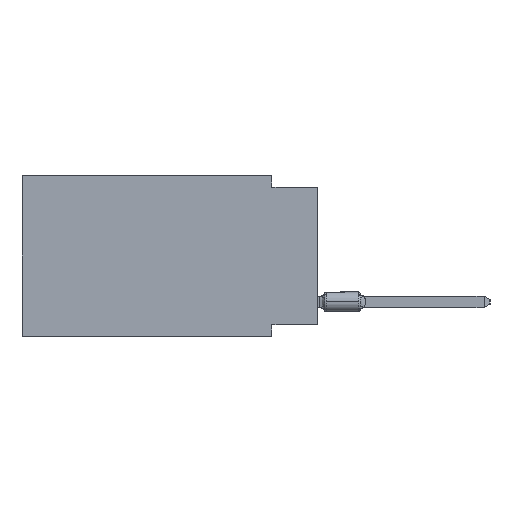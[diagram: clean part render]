
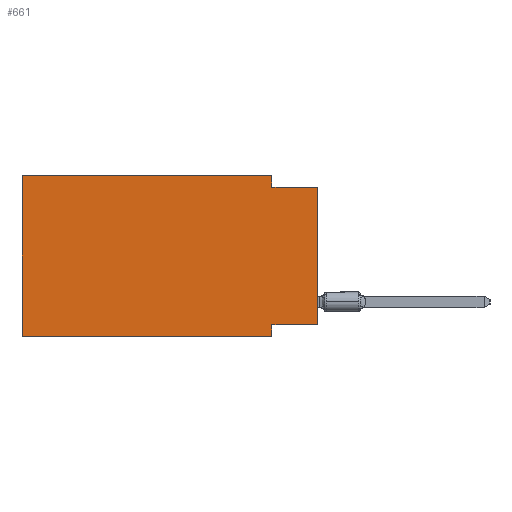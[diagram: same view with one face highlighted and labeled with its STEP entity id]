
A CAD part, left-side view. The second image highlights one B-rep face of the part: STEP entity #661.
In plain terms, the highlighted planar face has unit normal (-1, 0, 0).
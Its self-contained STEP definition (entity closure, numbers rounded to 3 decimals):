
#661 = ADVANCED_FACE ( 'NONE', ( #26702 ), #38116, .F. ) ;
#1163 = LINE ( 'NONE', #56208, #45565 ) ;
#1290 = VECTOR ( 'NONE', #16226, 1000. ) ;
#2733 = CARTESIAN_POINT ( 'NONE',  ( 0., 16.383, 0. ) ) ;
#2966 = CARTESIAN_POINT ( 'NONE',  ( 0., 16.383, 0. ) ) ;
#3619 = DIRECTION ( 'NONE',  ( 0., 0., 1. ) ) ;
#6558 = CARTESIAN_POINT ( 'NONE',  ( 0., 2.54, -0.635 ) ) ;
#6647 = LINE ( 'NONE', #50279, #53471 ) ;
#6813 = VERTEX_POINT ( 'NONE', #57139 ) ;
#7743 = LINE ( 'NONE', #2733, #22781 ) ;
#8327 = DIRECTION ( 'NONE',  ( 0., 1., 0. ) ) ;
#9110 = CARTESIAN_POINT ( 'NONE',  ( 0., 2.54, -8.89 ) ) ;
#10935 = CARTESIAN_POINT ( 'NONE',  ( 0., 16.383, -8.89 ) ) ;
#11896 = DIRECTION ( 'NONE',  ( 0., -1., 0. ) ) ;
#14308 = EDGE_CURVE ( 'NONE', #36126, #22864, #6647, .T. ) ;
#14360 = LINE ( 'NONE', #18653, #56139 ) ;
#15559 = ORIENTED_EDGE ( 'NONE', *, *, #39567, .T. ) ;
#16226 = DIRECTION ( 'NONE',  ( 0., 0., -1. ) ) ;
#17523 = DIRECTION ( 'NONE',  ( 0., -1., 0. ) ) ;
#18653 = CARTESIAN_POINT ( 'NONE',  ( 0., 0., 0. ) ) ;
#19734 = VERTEX_POINT ( 'NONE', #6558 ) ;
#22351 = ORIENTED_EDGE ( 'NONE', *, *, #59030, .F. ) ;
#22781 = VECTOR ( 'NONE', #51377, 1000. ) ;
#22864 = VERTEX_POINT ( 'NONE', #53963 ) ;
#24146 = LINE ( 'NONE', #9110, #40684 ) ;
#25913 = ORIENTED_EDGE ( 'NONE', *, *, #14308, .F. ) ;
#26702 = FACE_OUTER_BOUND ( 'NONE', #52631, .T. ) ;
#27064 = DIRECTION ( 'NONE',  ( 1., 0., 0. ) ) ;
#27695 = VECTOR ( 'NONE', #17523, 1000. ) ;
#33277 = EDGE_CURVE ( 'NONE', #45503, #19734, #37666, .T. ) ;
#34432 = EDGE_CURVE ( 'NONE', #19734, #68652, #45371, .T. ) ;
#35221 = VECTOR ( 'NONE', #68002, 1000. ) ;
#36126 = VERTEX_POINT ( 'NONE', #48187 ) ;
#37666 = LINE ( 'NONE', #59477, #1290 ) ;
#38116 = PLANE ( 'NONE',  #54300 ) ;
#39567 = EDGE_CURVE ( 'NONE', #36126, #68652, #14360, .T. ) ;
#40015 = CARTESIAN_POINT ( 'NONE',  ( 0., 0., -0.635 ) ) ;
#40684 = VECTOR ( 'NONE', #52740, 1000. ) ;
#41802 = ORIENTED_EDGE ( 'NONE', *, *, #64029, .F. ) ;
#45052 = VERTEX_POINT ( 'NONE', #2966 ) ;
#45121 = CARTESIAN_POINT ( 'NONE',  ( 0., 16.383, -8.89 ) ) ;
#45371 = LINE ( 'NONE', #40015, #27695 ) ;
#45503 = VERTEX_POINT ( 'NONE', #69888 ) ;
#45565 = VECTOR ( 'NONE', #11896, 1000. ) ;
#47772 = CARTESIAN_POINT ( 'NONE',  ( 0., 16.383, 0. ) ) ;
#48187 = CARTESIAN_POINT ( 'NONE',  ( 0., 0., -8.255 ) ) ;
#48429 = ORIENTED_EDGE ( 'NONE', *, *, #34432, .F. ) ;
#50279 = CARTESIAN_POINT ( 'NONE',  ( 0., 0., -8.255 ) ) ;
#51377 = DIRECTION ( 'NONE',  ( 0., 0., 1. ) ) ;
#52631 = EDGE_LOOP ( 'NONE', ( #15559, #48429, #59834, #41802, #62624, #70351, #22351, #25913 ) ) ;
#52740 = DIRECTION ( 'NONE',  ( 0., 0., -1. ) ) ;
#53471 = VECTOR ( 'NONE', #8327, 1000. ) ;
#53963 = CARTESIAN_POINT ( 'NONE',  ( 0., 2.54, -8.255 ) ) ;
#54300 = AXIS2_PLACEMENT_3D ( 'NONE', #47772, #27064, #65313 ) ;
#56139 = VECTOR ( 'NONE', #3619, 1000. ) ;
#56197 = CARTESIAN_POINT ( 'NONE',  ( 0., 0., -0.635 ) ) ;
#56208 = CARTESIAN_POINT ( 'NONE',  ( 0., 16.383, 0. ) ) ;
#57139 = CARTESIAN_POINT ( 'NONE',  ( 0., 2.54, -8.89 ) ) ;
#59030 = EDGE_CURVE ( 'NONE', #22864, #6813, #24146, .T. ) ;
#59477 = CARTESIAN_POINT ( 'NONE',  ( 0., 2.54, 0. ) ) ;
#59834 = ORIENTED_EDGE ( 'NONE', *, *, #33277, .F. ) ;
#62273 = LINE ( 'NONE', #45121, #35221 ) ;
#62580 = EDGE_CURVE ( 'NONE', #63629, #45052, #7743, .T. ) ;
#62624 = ORIENTED_EDGE ( 'NONE', *, *, #62580, .F. ) ;
#63629 = VERTEX_POINT ( 'NONE', #10935 ) ;
#64029 = EDGE_CURVE ( 'NONE', #45052, #45503, #1163, .T. ) ;
#65313 = DIRECTION ( 'NONE',  ( 0., 0., -1. ) ) ;
#68002 = DIRECTION ( 'NONE',  ( 0., -1., 0. ) ) ;
#68652 = VERTEX_POINT ( 'NONE', #56197 ) ;
#69865 = EDGE_CURVE ( 'NONE', #63629, #6813, #62273, .T. ) ;
#69888 = CARTESIAN_POINT ( 'NONE',  ( 0., 2.54, 0. ) ) ;
#70351 = ORIENTED_EDGE ( 'NONE', *, *, #69865, .T. ) ;
